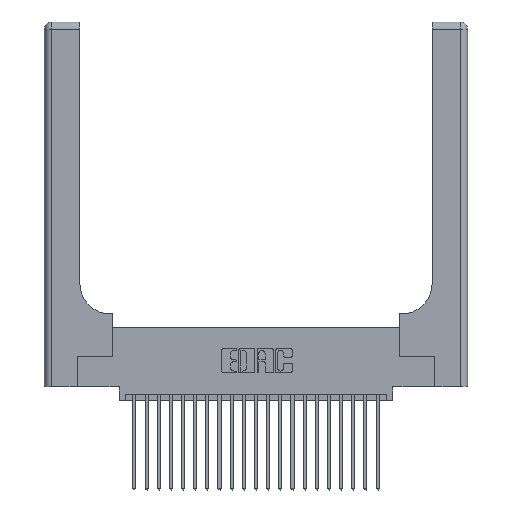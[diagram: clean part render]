
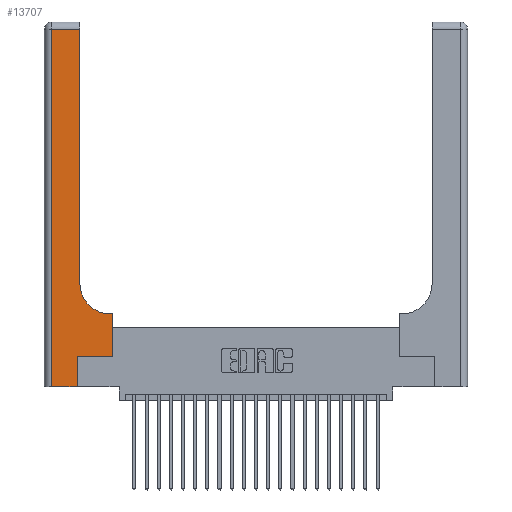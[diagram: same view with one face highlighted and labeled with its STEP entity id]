
A CAD part, top view. The second image highlights one B-rep face of the part: STEP entity #13707.
In plain terms, the highlighted planar face has unit normal (0, 0, 1).
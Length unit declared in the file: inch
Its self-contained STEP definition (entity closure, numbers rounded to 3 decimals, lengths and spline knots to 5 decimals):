
#567 = VERTEX_POINT ( 'NONE', #23405 ) ;
#615 = VECTOR ( 'NONE', #6241, 39.37008 ) ;
#792 = VERTEX_POINT ( 'NONE', #17567 ) ;
#1221 = VERTEX_POINT ( 'NONE', #20595 ) ;
#1330 = LINE ( 'NONE', #7976, #15451 ) ;
#1400 = ORIENTED_EDGE ( 'NONE', *, *, #14614, .T. ) ;
#1670 = DIRECTION ( 'NONE',  ( 0., 0., -1. ) ) ;
#1759 = LINE ( 'NONE', #10784, #6480 ) ;
#1880 = VERTEX_POINT ( 'NONE', #18665 ) ;
#1964 = ORIENTED_EDGE ( 'NONE', *, *, #23877, .T. ) ;
#2775 = CARTESIAN_POINT ( 'NONE',  ( 0.2915, 3., 0.37 ) ) ;
#3506 = DIRECTION ( 'NONE',  ( 0., -1., 0. ) ) ;
#3596 = EDGE_CURVE ( 'NONE', #1221, #792, #12590, .T. ) ;
#4435 = EDGE_CURVE ( 'NONE', #8745, #12499, #6667, .T. ) ;
#4810 = DIRECTION ( 'NONE',  ( 0., 1., 0. ) ) ;
#5135 = VERTEX_POINT ( 'NONE', #13371 ) ;
#5855 = VERTEX_POINT ( 'NONE', #15699 ) ;
#6059 = EDGE_LOOP ( 'NONE', ( #1964, #14272, #9776, #9554, #18007, #18581, #19269, #1400, #17783 ) ) ;
#6241 = DIRECTION ( 'NONE',  ( 1., 0., 0. ) ) ;
#6480 = VECTOR ( 'NONE', #14406, 39.37008 ) ;
#6667 = CIRCLE ( 'NONE', #8884, 0.25 ) ;
#7033 = EDGE_CURVE ( 'NONE', #15462, #1880, #19197, .T. ) ;
#7352 = LINE ( 'NONE', #18853, #21567 ) ;
#7616 = CARTESIAN_POINT ( 'NONE',  ( 0., 3., 0.37 ) ) ;
#7633 = VECTOR ( 'NONE', #23616, 39.37008 ) ;
#7714 = DIRECTION ( 'NONE',  ( 0., 0., -1. ) ) ;
#7976 = CARTESIAN_POINT ( 'NONE',  ( 0., 2.94, 0.37 ) ) ;
#8745 = VERTEX_POINT ( 'NONE', #14697 ) ;
#8884 = AXIS2_PLACEMENT_3D ( 'NONE', #18820, #7714, #20653 ) ;
#9554 = ORIENTED_EDGE ( 'NONE', *, *, #17513, .T. ) ;
#9776 = ORIENTED_EDGE ( 'NONE', *, *, #11934, .T. ) ;
#9892 = VECTOR ( 'NONE', #4810, 39.37008 ) ;
#10068 = FACE_OUTER_BOUND ( 'NONE', #6059, .T. ) ;
#10499 = LINE ( 'NONE', #15663, #615 ) ;
#10784 = CARTESIAN_POINT ( 'NONE',  ( 0.2915, 0.6, 0.37 ) ) ;
#11261 = CARTESIAN_POINT ( 'NONE',  ( 0.06, 3., 0.37 ) ) ;
#11934 = EDGE_CURVE ( 'NONE', #5855, #5135, #15824, .T. ) ;
#12499 = VERTEX_POINT ( 'NONE', #13125 ) ;
#12559 = EDGE_CURVE ( 'NONE', #792, #15462, #7352, .T. ) ;
#12590 = LINE ( 'NONE', #18063, #7633 ) ;
#12756 = AXIS2_PLACEMENT_3D ( 'NONE', #7616, #1670, #15093 ) ;
#13125 = CARTESIAN_POINT ( 'NONE',  ( 0.2915, 0.85, 0.37 ) ) ;
#13224 = PLANE ( 'NONE',  #12756 ) ;
#13371 = CARTESIAN_POINT ( 'NONE',  ( 0.06, 0., 0.37 ) ) ;
#13705 = VECTOR ( 'NONE', #24309, 39.37008 ) ;
#13707 = ADVANCED_FACE ( 'NONE', ( #10068 ), #13224, .F. ) ;
#14272 = ORIENTED_EDGE ( 'NONE', *, *, #16709, .T. ) ;
#14406 = DIRECTION ( 'NONE',  ( -1., 0., 0. ) ) ;
#14614 = EDGE_CURVE ( 'NONE', #1880, #8745, #1759, .T. ) ;
#14697 = CARTESIAN_POINT ( 'NONE',  ( 0.5415, 0.6, 0.37 ) ) ;
#15093 = DIRECTION ( 'NONE',  ( -1., 0., 0. ) ) ;
#15451 = VECTOR ( 'NONE', #17235, 39.37008 ) ;
#15462 = VERTEX_POINT ( 'NONE', #17133 ) ;
#15663 = CARTESIAN_POINT ( 'NONE',  ( 0., 0., 0.37 ) ) ;
#15699 = CARTESIAN_POINT ( 'NONE',  ( 0.06, 2.94, 0.37 ) ) ;
#15824 = LINE ( 'NONE', #11261, #20140 ) ;
#16709 = EDGE_CURVE ( 'NONE', #567, #5855, #1330, .T. ) ;
#17133 = CARTESIAN_POINT ( 'NONE',  ( 0.5585, 0.25, 0.37 ) ) ;
#17235 = DIRECTION ( 'NONE',  ( -1., 0., 0. ) ) ;
#17513 = EDGE_CURVE ( 'NONE', #5135, #1221, #10499, .T. ) ;
#17567 = CARTESIAN_POINT ( 'NONE',  ( 0.269, 0.25, 0.37 ) ) ;
#17783 = ORIENTED_EDGE ( 'NONE', *, *, #4435, .T. ) ;
#18007 = ORIENTED_EDGE ( 'NONE', *, *, #3596, .T. ) ;
#18063 = CARTESIAN_POINT ( 'NONE',  ( 0.269, 0., 0.37 ) ) ;
#18581 = ORIENTED_EDGE ( 'NONE', *, *, #12559, .T. ) ;
#18665 = CARTESIAN_POINT ( 'NONE',  ( 0.5585, 0.6, 0.37 ) ) ;
#18820 = CARTESIAN_POINT ( 'NONE',  ( 0.5415, 0.85, 0.37 ) ) ;
#18853 = CARTESIAN_POINT ( 'NONE',  ( 0.269, 0.25, 0.37 ) ) ;
#19197 = LINE ( 'NONE', #22419, #13705 ) ;
#19269 = ORIENTED_EDGE ( 'NONE', *, *, #7033, .T. ) ;
#19692 = LINE ( 'NONE', #2775, #9892 ) ;
#20140 = VECTOR ( 'NONE', #3506, 39.37008 ) ;
#20595 = CARTESIAN_POINT ( 'NONE',  ( 0.269, 0., 0.37 ) ) ;
#20653 = DIRECTION ( 'NONE',  ( 1., 0., 0. ) ) ;
#20683 = DIRECTION ( 'NONE',  ( 1., 0., 0. ) ) ;
#21567 = VECTOR ( 'NONE', #20683, 39.37008 ) ;
#22419 = CARTESIAN_POINT ( 'NONE',  ( 0.5585, 0.25, 0.37 ) ) ;
#23405 = CARTESIAN_POINT ( 'NONE',  ( 0.2915, 2.94, 0.37 ) ) ;
#23616 = DIRECTION ( 'NONE',  ( 0., 1., 0. ) ) ;
#23877 = EDGE_CURVE ( 'NONE', #12499, #567, #19692, .T. ) ;
#24309 = DIRECTION ( 'NONE',  ( 0., 1., 0. ) ) ;
